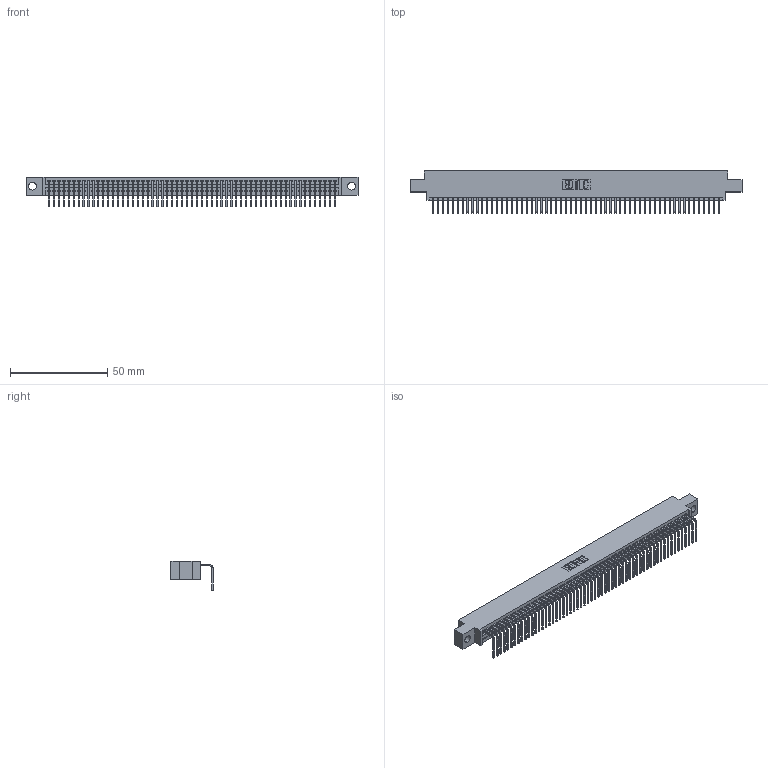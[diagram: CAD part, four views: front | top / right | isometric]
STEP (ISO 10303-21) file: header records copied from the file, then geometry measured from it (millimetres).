
FILE_DESCRIPTION (( 'STEP AP203' ), '1' );
FILE_NAME ('395-059-558-604.STEP', '2021-06-11T19:38:49', ( '' ), ( '' ), 'SwSTEP 2.0', 'SolidWorks 2020', '' );
FILE_SCHEMA (( 'CONFIG_CONTROL_DESIGN' ));
Length unit declared in the file: inch
Products named in the file (3): 395-059-558-604; 345-292-001_558 Tail - 2; 345 Part_0.170 Offset - 0.156 Dia-TI
Assembly tree (60 placements, depth 2):
  395-059-558-604
    345 Part_0.170 Offset - 0.156 Dia-TI
    345-292-001_558 Tail - 2  x59
Bounding box: 171.07 x 21.83 x 15.37 mm (x, y, z)
Volume: 16364.8 mm3; surface area: 23102.5 mm2
Topology: 60 solids, 60 shells, 3684 faces, 11127 edges, 7338 vertices
Faces by surface type: plane 2576, cylinder 1108
Entity records: 42751 total; most frequent: CARTESIAN_POINT 7415, ORIENTED_EDGE 7406, DIRECTION 6449, EDGE_CURVE 3703, VECTOR 3335, LINE 3335, VERTEX_POINT 2466, AXIS2_PLACEMENT_3D 1557
